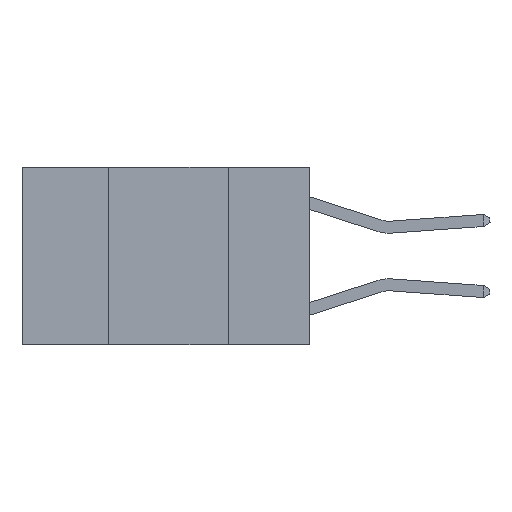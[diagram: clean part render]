
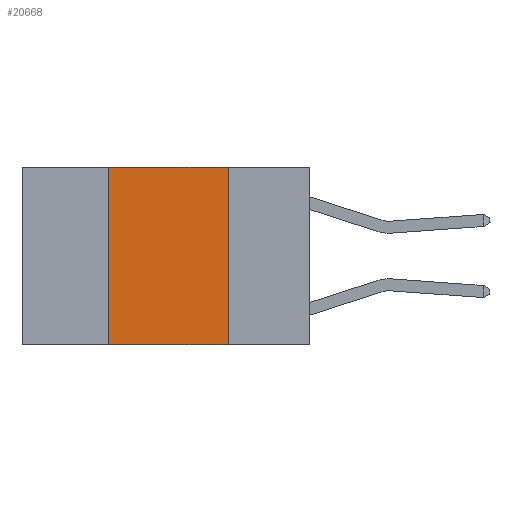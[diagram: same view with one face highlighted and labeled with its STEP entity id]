
A CAD part, left-side view. The second image highlights one B-rep face of the part: STEP entity #20668.
In plain terms, the highlighted planar face has unit normal (-1, 0, 0).
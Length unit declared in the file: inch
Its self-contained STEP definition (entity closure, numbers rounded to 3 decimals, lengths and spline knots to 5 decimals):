
#22 = DIRECTION ( 'NONE',  ( 0., -1., 0. ) ) ;
#31 = ORIENTED_EDGE ( 'NONE', *, *, #13777, .F. ) ;
#512 = CARTESIAN_POINT ( 'NONE',  ( 0., 0.42, 0. ) ) ;
#579 = EDGE_CURVE ( 'NONE', #3823, #19933, #16291, .T. ) ;
#1099 = LINE ( 'NONE', #7315, #3409 ) ;
#1883 = CARTESIAN_POINT ( 'NONE',  ( 0., 0.6, 0. ) ) ;
#1927 = VERTEX_POINT ( 'NONE', #16427 ) ;
#3409 = VECTOR ( 'NONE', #7528, 39.37008 ) ;
#3823 = VERTEX_POINT ( 'NONE', #512 ) ;
#4038 = VECTOR ( 'NONE', #15094, 39.37008 ) ;
#4664 = CARTESIAN_POINT ( 'NONE',  ( 0., 0.6, -0.37 ) ) ;
#5033 = EDGE_CURVE ( 'NONE', #1927, #14090, #19298, .T. ) ;
#5685 = CARTESIAN_POINT ( 'NONE',  ( 0., 0.17, 0. ) ) ;
#6393 = DIRECTION ( 'NONE',  ( 0., 0., -1. ) ) ;
#7315 = CARTESIAN_POINT ( 'NONE',  ( 0., 0.42, 0. ) ) ;
#7528 = DIRECTION ( 'NONE',  ( 0., 0., 1. ) ) ;
#8208 = DIRECTION ( 'NONE',  ( 0., -1., 0. ) ) ;
#9564 = EDGE_LOOP ( 'NONE', ( #31, #18191, #16574, #14245 ) ) ;
#9688 = PLANE ( 'NONE',  #15301 ) ;
#10038 = CARTESIAN_POINT ( 'NONE',  ( 0., 0.17, -0.37 ) ) ;
#11252 = CARTESIAN_POINT ( 'NONE',  ( 0., 0.6, 0. ) ) ;
#11362 = FACE_OUTER_BOUND ( 'NONE', #9564, .T. ) ;
#11718 = VECTOR ( 'NONE', #8208, 39.37008 ) ;
#12083 = VECTOR ( 'NONE', #22, 39.37008 ) ;
#13777 = EDGE_CURVE ( 'NONE', #19933, #14090, #16752, .T. ) ;
#14090 = VERTEX_POINT ( 'NONE', #10038 ) ;
#14245 = ORIENTED_EDGE ( 'NONE', *, *, #5033, .T. ) ;
#14375 = DIRECTION ( 'NONE',  ( 1., 0., 0. ) ) ;
#14706 = EDGE_CURVE ( 'NONE', #1927, #3823, #1099, .T. ) ;
#15094 = DIRECTION ( 'NONE',  ( 0., 0., -1. ) ) ;
#15301 = AXIS2_PLACEMENT_3D ( 'NONE', #11252, #14375, #6393 ) ;
#16291 = LINE ( 'NONE', #1883, #11718 ) ;
#16427 = CARTESIAN_POINT ( 'NONE',  ( 0., 0.42, -0.37 ) ) ;
#16574 = ORIENTED_EDGE ( 'NONE', *, *, #14706, .F. ) ;
#16752 = LINE ( 'NONE', #5685, #4038 ) ;
#18165 = CARTESIAN_POINT ( 'NONE',  ( 0., 0.17, 0. ) ) ;
#18191 = ORIENTED_EDGE ( 'NONE', *, *, #579, .F. ) ;
#19298 = LINE ( 'NONE', #4664, #12083 ) ;
#19933 = VERTEX_POINT ( 'NONE', #18165 ) ;
#20668 = ADVANCED_FACE ( 'NONE', ( #11362 ), #9688, .F. ) ;
